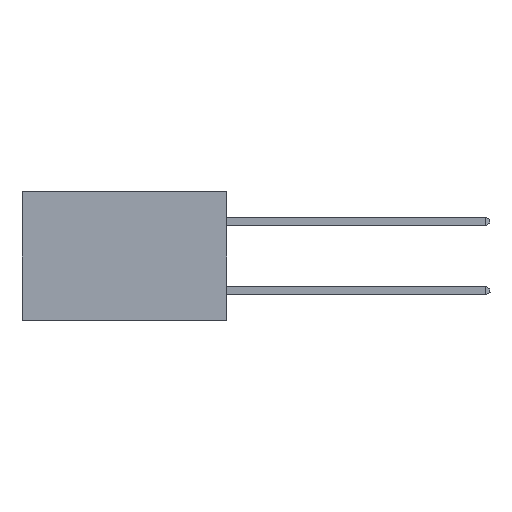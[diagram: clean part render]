
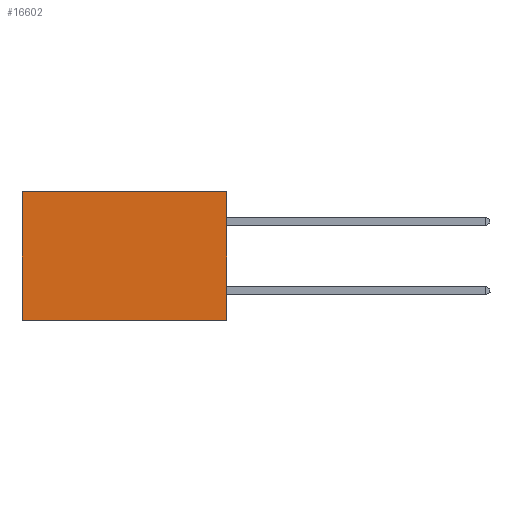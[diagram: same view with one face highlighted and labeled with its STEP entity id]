
A CAD part, left-side view. The second image highlights one B-rep face of the part: STEP entity #16602.
In plain terms, the highlighted planar face has unit normal (-1, 0, 0).
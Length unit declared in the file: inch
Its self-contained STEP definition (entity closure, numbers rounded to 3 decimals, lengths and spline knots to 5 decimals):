
#166 = VECTOR ( 'NONE', #924, 39.37008 ) ;
#574 = ORIENTED_EDGE ( 'NONE', *, *, #30168, .T. ) ;
#924 = DIRECTION ( 'NONE',  ( 0., 0., -1. ) ) ;
#3203 = VECTOR ( 'NONE', #28925, 39.37008 ) ;
#4376 = CARTESIAN_POINT ( 'NONE',  ( 0.277, 0.59, -0.37 ) ) ;
#4460 = CARTESIAN_POINT ( 'NONE',  ( 0.277, 0., -0.37 ) ) ;
#4650 = CARTESIAN_POINT ( 'NONE',  ( 0.277, 0.59, -0.37 ) ) ;
#4747 = EDGE_CURVE ( 'NONE', #15499, #19433, #30085, .T. ) ;
#4840 = CARTESIAN_POINT ( 'NONE',  ( 0.277, 0., -0.37 ) ) ;
#5637 = CARTESIAN_POINT ( 'NONE',  ( 0.277, 0., 0. ) ) ;
#6226 = LINE ( 'NONE', #4376, #17141 ) ;
#6304 = AXIS2_PLACEMENT_3D ( 'NONE', #4460, #12074, #29425 ) ;
#9940 = LINE ( 'NONE', #26424, #3203 ) ;
#10885 = EDGE_CURVE ( 'NONE', #25586, #19939, #9940, .T. ) ;
#11132 = DIRECTION ( 'NONE',  ( 0., 1., 0. ) ) ;
#11267 = CARTESIAN_POINT ( 'NONE',  ( 0.277, 0., 0. ) ) ;
#12074 = DIRECTION ( 'NONE',  ( 1., 0., 0. ) ) ;
#14144 = ORIENTED_EDGE ( 'NONE', *, *, #4747, .T. ) ;
#15499 = VERTEX_POINT ( 'NONE', #5637 ) ;
#16602 = ADVANCED_FACE ( 'NONE', ( #22741 ), #29223, .F. ) ;
#17141 = VECTOR ( 'NONE', #24357, 39.37008 ) ;
#17849 = ORIENTED_EDGE ( 'NONE', *, *, #10885, .F. ) ;
#19433 = VERTEX_POINT ( 'NONE', #27264 ) ;
#19939 = VERTEX_POINT ( 'NONE', #4650 ) ;
#20171 = LINE ( 'NONE', #30829, #166 ) ;
#22741 = FACE_OUTER_BOUND ( 'NONE', #24726, .T. ) ;
#23020 = ORIENTED_EDGE ( 'NONE', *, *, #31400, .F. ) ;
#23495 = VECTOR ( 'NONE', #11132, 39.37008 ) ;
#24357 = DIRECTION ( 'NONE',  ( 0., 0., -1. ) ) ;
#24726 = EDGE_LOOP ( 'NONE', ( #574, #17849, #23020, #14144 ) ) ;
#25586 = VERTEX_POINT ( 'NONE', #4840 ) ;
#26424 = CARTESIAN_POINT ( 'NONE',  ( 0.277, 0., -0.37 ) ) ;
#27264 = CARTESIAN_POINT ( 'NONE',  ( 0.277, 0.59, 0. ) ) ;
#28925 = DIRECTION ( 'NONE',  ( 0., 1., 0. ) ) ;
#29223 = PLANE ( 'NONE',  #6304 ) ;
#29425 = DIRECTION ( 'NONE',  ( 0., 0., -1. ) ) ;
#30085 = LINE ( 'NONE', #11267, #23495 ) ;
#30168 = EDGE_CURVE ( 'NONE', #19433, #19939, #6226, .T. ) ;
#30829 = CARTESIAN_POINT ( 'NONE',  ( 0.277, 0., -0.37 ) ) ;
#31400 = EDGE_CURVE ( 'NONE', #15499, #25586, #20171, .T. ) ;
